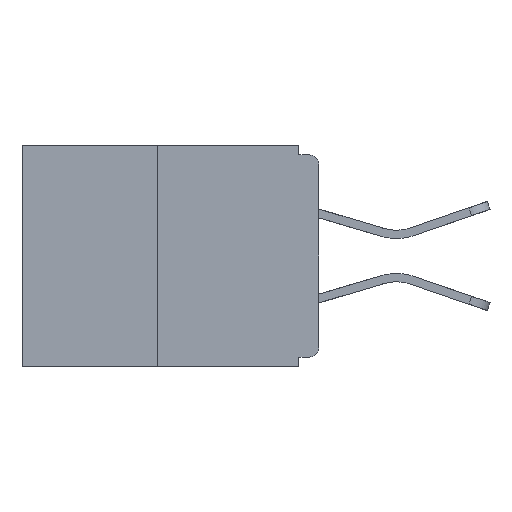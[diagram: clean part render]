
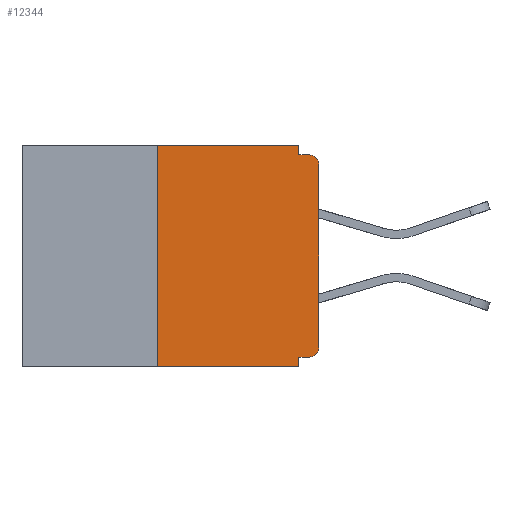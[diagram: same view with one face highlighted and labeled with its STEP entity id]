
A CAD part, left-side view. The second image highlights one B-rep face of the part: STEP entity #12344.
In plain terms, the highlighted planar face has unit normal (-1, 0, 0).
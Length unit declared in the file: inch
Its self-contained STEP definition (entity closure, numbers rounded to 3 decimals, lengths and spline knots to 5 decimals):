
#43 = VECTOR ( 'NONE', #11716, 39.37008 ) ;
#251 = CARTESIAN_POINT ( 'NONE',  ( 0., 0.25, -0.343 ) ) ;
#591 = DIRECTION ( 'NONE',  ( 0., 0., -1. ) ) ;
#839 = VERTEX_POINT ( 'NONE', #1910 ) ;
#1086 = CARTESIAN_POINT ( 'NONE',  ( 0., 0.25, 0. ) ) ;
#1199 = ORIENTED_EDGE ( 'NONE', *, *, #16222, .F. ) ;
#1698 = DIRECTION ( 'NONE',  ( -1., 0., 0. ) ) ;
#1910 = CARTESIAN_POINT ( 'NONE',  ( 0., 0.015, -0.015 ) ) ;
#2452 = CARTESIAN_POINT ( 'NONE',  ( 0., 0., -0.015 ) ) ;
#2700 = CARTESIAN_POINT ( 'NONE',  ( 0., 0., -0.313 ) ) ;
#2952 = ORIENTED_EDGE ( 'NONE', *, *, #20850, .F. ) ;
#3063 = ORIENTED_EDGE ( 'NONE', *, *, #14165, .F. ) ;
#3212 = CARTESIAN_POINT ( 'NONE',  ( 0., 0., -0.03 ) ) ;
#3486 = VERTEX_POINT ( 'NONE', #251 ) ;
#3534 = EDGE_CURVE ( 'NONE', #21998, #15200, #12624, .T. ) ;
#3718 = AXIS2_PLACEMENT_3D ( 'NONE', #23993, #1698, #21894 ) ;
#4552 = DIRECTION ( 'NONE',  ( 1., 0., 0. ) ) ;
#5361 = LINE ( 'NONE', #1086, #13238 ) ;
#6262 = DIRECTION ( 'NONE',  ( 0., -1., 0. ) ) ;
#6408 = EDGE_CURVE ( 'NONE', #10744, #8065, #9018, .T. ) ;
#6659 = AXIS2_PLACEMENT_3D ( 'NONE', #9993, #23067, #591 ) ;
#6952 = CIRCLE ( 'NONE', #3718, 0.015 ) ;
#6991 = CARTESIAN_POINT ( 'NONE',  ( 0., 0., -0.328 ) ) ;
#7371 = EDGE_CURVE ( 'NONE', #12640, #839, #14592, .T. ) ;
#7401 = VECTOR ( 'NONE', #7545, 39.37008 ) ;
#7483 = EDGE_CURVE ( 'NONE', #3486, #8065, #16059, .T. ) ;
#7545 = DIRECTION ( 'NONE',  ( 0., 0., 1. ) ) ;
#8065 = VERTEX_POINT ( 'NONE', #11260 ) ;
#8082 = CARTESIAN_POINT ( 'NONE',  ( 0., 0.031, -0.343 ) ) ;
#8318 = DIRECTION ( 'NONE',  ( 0., 0., -1. ) ) ;
#9018 = LINE ( 'NONE', #8082, #12803 ) ;
#9081 = CARTESIAN_POINT ( 'NONE',  ( 0., 0.031, -0.015 ) ) ;
#9779 = ORIENTED_EDGE ( 'NONE', *, *, #6408, .F. ) ;
#9993 = CARTESIAN_POINT ( 'NONE',  ( 0., 0.015, -0.313 ) ) ;
#10215 = EDGE_CURVE ( 'NONE', #11811, #839, #6952, .T. ) ;
#10732 = LINE ( 'NONE', #6991, #11911 ) ;
#10744 = VERTEX_POINT ( 'NONE', #13696 ) ;
#10858 = FACE_OUTER_BOUND ( 'NONE', #13988, .T. ) ;
#11260 = CARTESIAN_POINT ( 'NONE',  ( 0., 0.031, -0.343 ) ) ;
#11716 = DIRECTION ( 'NONE',  ( 0., -1., 0. ) ) ;
#11811 = VERTEX_POINT ( 'NONE', #3212 ) ;
#11911 = VECTOR ( 'NONE', #14452, 39.37008 ) ;
#12344 = ADVANCED_FACE ( 'NONE', ( #10858 ), #13952, .F. ) ;
#12366 = CARTESIAN_POINT ( 'NONE',  ( 0., 0.031, 0. ) ) ;
#12624 = CIRCLE ( 'NONE', #6659, 0.015 ) ;
#12640 = VERTEX_POINT ( 'NONE', #9081 ) ;
#12803 = VECTOR ( 'NONE', #23008, 39.37008 ) ;
#12965 = CARTESIAN_POINT ( 'NONE',  ( 0., 0.031, 0. ) ) ;
#12987 = ORIENTED_EDGE ( 'NONE', *, *, #7483, .T. ) ;
#13238 = VECTOR ( 'NONE', #23392, 39.37008 ) ;
#13335 = DIRECTION ( 'NONE',  ( 0., -1., 0. ) ) ;
#13347 = CARTESIAN_POINT ( 'NONE',  ( 0., 0.25, 0. ) ) ;
#13696 = CARTESIAN_POINT ( 'NONE',  ( 0., 0.031, -0.328 ) ) ;
#13699 = CARTESIAN_POINT ( 'NONE',  ( 0., 0.46, 0. ) ) ;
#13880 = LINE ( 'NONE', #18680, #7401 ) ;
#13952 = PLANE ( 'NONE',  #19850 ) ;
#13988 = EDGE_LOOP ( 'NONE', ( #2952, #1199, #12987, #9779, #3063, #22064, #20516, #16039, #18687, #16470 ) ) ;
#14165 = EDGE_CURVE ( 'NONE', #21998, #10744, #10732, .T. ) ;
#14452 = DIRECTION ( 'NONE',  ( 0., 1., 0. ) ) ;
#14592 = LINE ( 'NONE', #2452, #22662 ) ;
#14719 = LINE ( 'NONE', #12366, #19081 ) ;
#15200 = VERTEX_POINT ( 'NONE', #2700 ) ;
#15796 = CARTESIAN_POINT ( 'NONE',  ( 0., 0.46, 0. ) ) ;
#15863 = EDGE_CURVE ( 'NONE', #16948, #12640, #14719, .T. ) ;
#16039 = ORIENTED_EDGE ( 'NONE', *, *, #10215, .T. ) ;
#16059 = LINE ( 'NONE', #19590, #16903 ) ;
#16222 = EDGE_CURVE ( 'NONE', #3486, #23865, #5361, .T. ) ;
#16470 = ORIENTED_EDGE ( 'NONE', *, *, #15863, .F. ) ;
#16886 = CARTESIAN_POINT ( 'NONE',  ( 0., 0.015, -0.328 ) ) ;
#16903 = VECTOR ( 'NONE', #6262, 39.37008 ) ;
#16948 = VERTEX_POINT ( 'NONE', #12965 ) ;
#18121 = DIRECTION ( 'NONE',  ( 0., 0., -1. ) ) ;
#18680 = CARTESIAN_POINT ( 'NONE',  ( 0., 0., 0. ) ) ;
#18687 = ORIENTED_EDGE ( 'NONE', *, *, #7371, .F. ) ;
#19081 = VECTOR ( 'NONE', #18121, 39.37008 ) ;
#19499 = EDGE_CURVE ( 'NONE', #15200, #11811, #13880, .T. ) ;
#19590 = CARTESIAN_POINT ( 'NONE',  ( 0., 0.46, -0.343 ) ) ;
#19850 = AXIS2_PLACEMENT_3D ( 'NONE', #15796, #4552, #8318 ) ;
#20516 = ORIENTED_EDGE ( 'NONE', *, *, #19499, .T. ) ;
#20850 = EDGE_CURVE ( 'NONE', #23865, #16948, #23738, .T. ) ;
#21894 = DIRECTION ( 'NONE',  ( 0., 0., -1. ) ) ;
#21998 = VERTEX_POINT ( 'NONE', #16886 ) ;
#22064 = ORIENTED_EDGE ( 'NONE', *, *, #3534, .T. ) ;
#22662 = VECTOR ( 'NONE', #13335, 39.37008 ) ;
#23008 = DIRECTION ( 'NONE',  ( 0., 0., -1. ) ) ;
#23067 = DIRECTION ( 'NONE',  ( -1., 0., 0. ) ) ;
#23392 = DIRECTION ( 'NONE',  ( 0., 0., 1. ) ) ;
#23738 = LINE ( 'NONE', #13699, #43 ) ;
#23865 = VERTEX_POINT ( 'NONE', #13347 ) ;
#23993 = CARTESIAN_POINT ( 'NONE',  ( 0., 0.015, -0.03 ) ) ;
